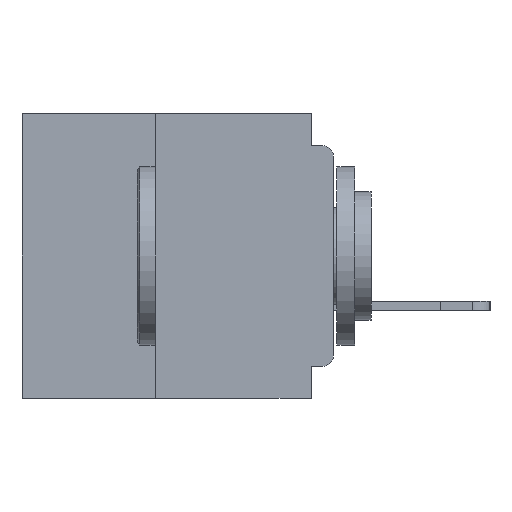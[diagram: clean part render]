
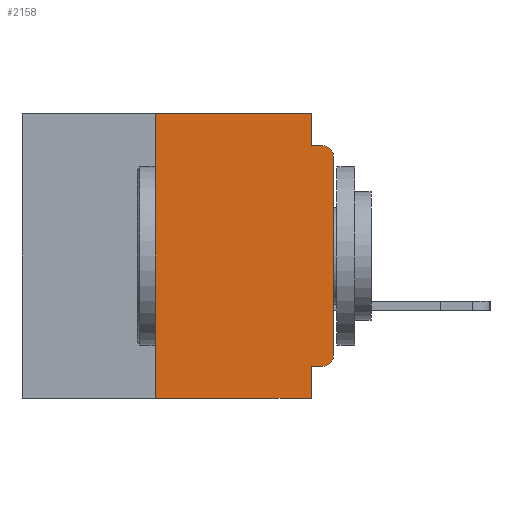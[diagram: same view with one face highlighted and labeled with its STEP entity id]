
A CAD part, left-side view. The second image highlights one B-rep face of the part: STEP entity #2158.
In plain terms, the highlighted planar face has unit normal (-1, 0, 0).
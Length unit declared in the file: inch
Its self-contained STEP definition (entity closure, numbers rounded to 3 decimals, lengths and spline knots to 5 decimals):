
#743 = ORIENTED_EDGE ( 'NONE', *, *, #5093, .T. ) ;
#947 = LINE ( 'NONE', #38794, #37580 ) ;
#965 = CARTESIAN_POINT ( 'NONE',  ( 0., 0.031, -0.4 ) ) ;
#1693 = EDGE_CURVE ( 'NONE', #46353, #38919, #23451, .T. ) ;
#1705 = LINE ( 'NONE', #21305, #20058 ) ;
#2158 = ADVANCED_FACE ( 'NONE', ( #12579 ), #36517, .F. ) ;
#3479 = CARTESIAN_POINT ( 'NONE',  ( 0., 0., -0.06 ) ) ;
#3598 = ORIENTED_EDGE ( 'NONE', *, *, #5231, .F. ) ;
#4751 = AXIS2_PLACEMENT_3D ( 'NONE', #37256, #36306, #36244 ) ;
#5093 = EDGE_CURVE ( 'NONE', #38919, #8536, #15370, .T. ) ;
#5195 = CARTESIAN_POINT ( 'NONE',  ( 0., 0.031, -0.4 ) ) ;
#5231 = EDGE_CURVE ( 'NONE', #36693, #8536, #7337, .T. ) ;
#6752 = DIRECTION ( 'NONE',  ( 0., 0., -1. ) ) ;
#7337 = LINE ( 'NONE', #29441, #35349 ) ;
#8112 = LINE ( 'NONE', #34950, #45877 ) ;
#8172 = CARTESIAN_POINT ( 'NONE',  ( 0., 0.031, 0. ) ) ;
#8536 = VERTEX_POINT ( 'NONE', #34166 ) ;
#9225 = EDGE_CURVE ( 'NONE', #28032, #31206, #23543, .T. ) ;
#10544 = DIRECTION ( 'NONE',  ( -1., 0., 0. ) ) ;
#12170 = EDGE_CURVE ( 'NONE', #31754, #36693, #1705, .T. ) ;
#12579 = FACE_OUTER_BOUND ( 'NONE', #28292, .T. ) ;
#13550 = CARTESIAN_POINT ( 'NONE',  ( 0., 0.437, -0.4 ) ) ;
#13769 = VECTOR ( 'NONE', #38702, 39.37008 ) ;
#14198 = CARTESIAN_POINT ( 'NONE',  ( 0., 0.015, -0.34 ) ) ;
#14996 = DIRECTION ( 'NONE',  ( 0., -1., 0. ) ) ;
#15370 = CIRCLE ( 'NONE', #30780, 0.015 ) ;
#15825 = ORIENTED_EDGE ( 'NONE', *, *, #35474, .F. ) ;
#16709 = CARTESIAN_POINT ( 'NONE',  ( 0., 0., -0.34 ) ) ;
#17254 = DIRECTION ( 'NONE',  ( 0., -1., 0. ) ) ;
#17602 = ORIENTED_EDGE ( 'NONE', *, *, #45147, .F. ) ;
#17915 = DIRECTION ( 'NONE',  ( 0., 0., -1. ) ) ;
#17961 = EDGE_CURVE ( 'NONE', #33349, #43516, #8112, .T. ) ;
#18175 = CARTESIAN_POINT ( 'NONE',  ( 0., 0.015, -0.355 ) ) ;
#20058 = VECTOR ( 'NONE', #6752, 39.37008 ) ;
#20587 = DIRECTION ( 'NONE',  ( 0., -1., 0. ) ) ;
#20737 = CARTESIAN_POINT ( 'NONE',  ( 0., 0.25, -0.4 ) ) ;
#21298 = VECTOR ( 'NONE', #17254, 39.37008 ) ;
#21305 = CARTESIAN_POINT ( 'NONE',  ( 0., 0.031, 0. ) ) ;
#21517 = ORIENTED_EDGE ( 'NONE', *, *, #1693, .T. ) ;
#23451 = LINE ( 'NONE', #38073, #13769 ) ;
#23543 = LINE ( 'NONE', #13550, #21298 ) ;
#24861 = CARTESIAN_POINT ( 'NONE',  ( 0., 0.031, -0.045 ) ) ;
#25306 = EDGE_CURVE ( 'NONE', #33349, #46353, #33092, .T. ) ;
#25445 = CARTESIAN_POINT ( 'NONE',  ( 0., 0.25, -0.4 ) ) ;
#25530 = ORIENTED_EDGE ( 'NONE', *, *, #12170, .F. ) ;
#26361 = LINE ( 'NONE', #965, #37261 ) ;
#26520 = DIRECTION ( 'NONE',  ( 0., 0., -1. ) ) ;
#27896 = AXIS2_PLACEMENT_3D ( 'NONE', #14198, #39755, #17915 ) ;
#28032 = VERTEX_POINT ( 'NONE', #20737 ) ;
#28175 = VERTEX_POINT ( 'NONE', #32496 ) ;
#28292 = EDGE_LOOP ( 'NONE', ( #21517, #743, #3598, #25530, #17602, #15825, #40129, #34658, #29869, #42841 ) ) ;
#29074 = DIRECTION ( 'NONE',  ( 0., 0., 1. ) ) ;
#29441 = CARTESIAN_POINT ( 'NONE',  ( 0., 0., -0.045 ) ) ;
#29869 = ORIENTED_EDGE ( 'NONE', *, *, #17961, .F. ) ;
#30780 = AXIS2_PLACEMENT_3D ( 'NONE', #32351, #10544, #36096 ) ;
#31206 = VERTEX_POINT ( 'NONE', #5195 ) ;
#31754 = VERTEX_POINT ( 'NONE', #8172 ) ;
#32351 = CARTESIAN_POINT ( 'NONE',  ( 0., 0.015, -0.06 ) ) ;
#32496 = CARTESIAN_POINT ( 'NONE',  ( 0., 0.25, 0. ) ) ;
#33092 = CIRCLE ( 'NONE', #27896, 0.015 ) ;
#33349 = VERTEX_POINT ( 'NONE', #18175 ) ;
#34166 = CARTESIAN_POINT ( 'NONE',  ( 0., 0.015, -0.045 ) ) ;
#34658 = ORIENTED_EDGE ( 'NONE', *, *, #35638, .F. ) ;
#34950 = CARTESIAN_POINT ( 'NONE',  ( 0., 0., -0.355 ) ) ;
#35120 = DIRECTION ( 'NONE',  ( 0., 1., 0. ) ) ;
#35349 = VECTOR ( 'NONE', #14996, 39.37008 ) ;
#35474 = EDGE_CURVE ( 'NONE', #28032, #28175, #35587, .T. ) ;
#35587 = LINE ( 'NONE', #25445, #44164 ) ;
#35638 = EDGE_CURVE ( 'NONE', #43516, #31206, #26361, .T. ) ;
#35748 = CARTESIAN_POINT ( 'NONE',  ( 0., 0.031, -0.355 ) ) ;
#36096 = DIRECTION ( 'NONE',  ( 0., 0., -1. ) ) ;
#36244 = DIRECTION ( 'NONE',  ( 0., 0., -1. ) ) ;
#36306 = DIRECTION ( 'NONE',  ( 1., 0., 0. ) ) ;
#36517 = PLANE ( 'NONE',  #4751 ) ;
#36693 = VERTEX_POINT ( 'NONE', #24861 ) ;
#37256 = CARTESIAN_POINT ( 'NONE',  ( 0., 0.437, 0. ) ) ;
#37261 = VECTOR ( 'NONE', #26520, 39.37008 ) ;
#37580 = VECTOR ( 'NONE', #20587, 39.37008 ) ;
#38073 = CARTESIAN_POINT ( 'NONE',  ( 0., 0., 0. ) ) ;
#38702 = DIRECTION ( 'NONE',  ( 0., 0., 1. ) ) ;
#38794 = CARTESIAN_POINT ( 'NONE',  ( 0., 0.437, 0. ) ) ;
#38919 = VERTEX_POINT ( 'NONE', #3479 ) ;
#39755 = DIRECTION ( 'NONE',  ( -1., 0., 0. ) ) ;
#40129 = ORIENTED_EDGE ( 'NONE', *, *, #9225, .T. ) ;
#42841 = ORIENTED_EDGE ( 'NONE', *, *, #25306, .T. ) ;
#43516 = VERTEX_POINT ( 'NONE', #35748 ) ;
#44164 = VECTOR ( 'NONE', #29074, 39.37008 ) ;
#45147 = EDGE_CURVE ( 'NONE', #28175, #31754, #947, .T. ) ;
#45877 = VECTOR ( 'NONE', #35120, 39.37008 ) ;
#46353 = VERTEX_POINT ( 'NONE', #16709 ) ;
